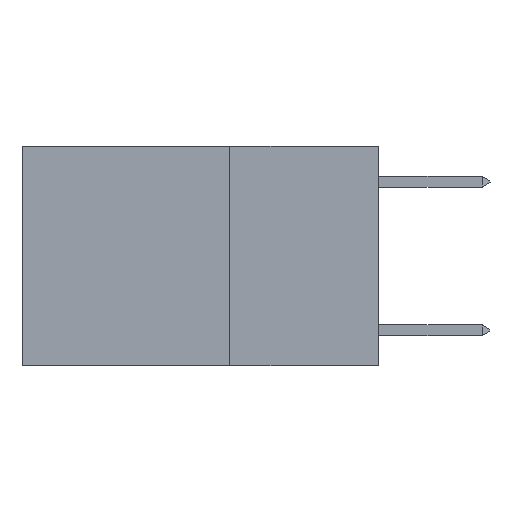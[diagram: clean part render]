
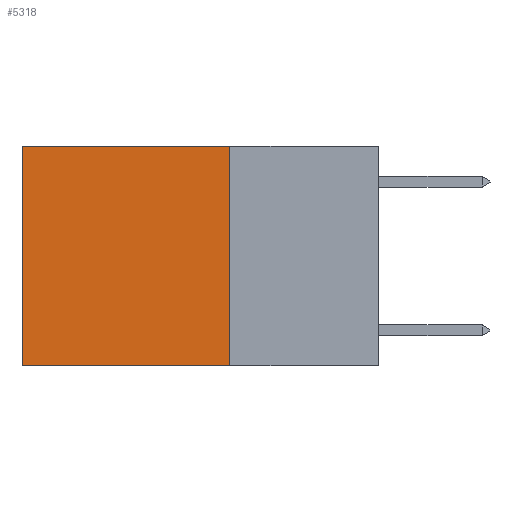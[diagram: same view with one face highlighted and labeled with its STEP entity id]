
A CAD part, left-side view. The second image highlights one B-rep face of the part: STEP entity #5318.
In plain terms, the highlighted planar face has unit normal (-1, 0, 0).
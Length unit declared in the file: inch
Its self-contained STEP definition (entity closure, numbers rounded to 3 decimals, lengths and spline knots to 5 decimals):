
#145 = CARTESIAN_POINT ( 'NONE',  ( 0.2625, 0.6, 0. ) ) ;
#377 = VERTEX_POINT ( 'NONE', #5765 ) ;
#476 = VECTOR ( 'NONE', #7910, 39.37008 ) ;
#865 = CARTESIAN_POINT ( 'NONE',  ( 0.2625, 0.25, 0. ) ) ;
#945 = DIRECTION ( 'NONE',  ( 1., 0., 0. ) ) ;
#957 = DIRECTION ( 'NONE',  ( 0., 1., 0. ) ) ;
#2212 = CARTESIAN_POINT ( 'NONE',  ( 0.2625, 0.6, -0.37 ) ) ;
#2438 = VERTEX_POINT ( 'NONE', #7295 ) ;
#2687 = VECTOR ( 'NONE', #13122, 39.37008 ) ;
#3317 = FACE_OUTER_BOUND ( 'NONE', #9579, .T. ) ;
#3550 = EDGE_CURVE ( 'NONE', #377, #9089, #14127, .T. ) ;
#3612 = ORIENTED_EDGE ( 'NONE', *, *, #13934, .F. ) ;
#4056 = CARTESIAN_POINT ( 'NONE',  ( 0.2625, 0.25, 0. ) ) ;
#4208 = VECTOR ( 'NONE', #7472, 39.37008 ) ;
#4523 = DIRECTION ( 'NONE',  ( 0., 0., -1. ) ) ;
#4984 = ORIENTED_EDGE ( 'NONE', *, *, #5076, .F. ) ;
#5076 = EDGE_CURVE ( 'NONE', #2438, #8968, #8443, .T. ) ;
#5084 = LINE ( 'NONE', #4056, #4208 ) ;
#5301 = CARTESIAN_POINT ( 'NONE',  ( 0.2625, 0.6, 0. ) ) ;
#5318 = ADVANCED_FACE ( 'NONE', ( #3317 ), #15074, .F. ) ;
#5765 = CARTESIAN_POINT ( 'NONE',  ( 0.2625, 0.25, 0. ) ) ;
#7229 = LINE ( 'NONE', #5301, #476 ) ;
#7295 = CARTESIAN_POINT ( 'NONE',  ( 0.2625, 0.25, -0.37 ) ) ;
#7472 = DIRECTION ( 'NONE',  ( 0., 0., -1. ) ) ;
#7910 = DIRECTION ( 'NONE',  ( 0., 0., -1. ) ) ;
#8443 = LINE ( 'NONE', #9407, #2687 ) ;
#8968 = VERTEX_POINT ( 'NONE', #2212 ) ;
#9089 = VERTEX_POINT ( 'NONE', #145 ) ;
#9269 = ORIENTED_EDGE ( 'NONE', *, *, #15321, .T. ) ;
#9407 = CARTESIAN_POINT ( 'NONE',  ( 0.2625, 0.25, -0.37 ) ) ;
#9579 = EDGE_LOOP ( 'NONE', ( #9269, #4984, #3612, #11274 ) ) ;
#11274 = ORIENTED_EDGE ( 'NONE', *, *, #3550, .T. ) ;
#11505 = AXIS2_PLACEMENT_3D ( 'NONE', #865, #945, #4523 ) ;
#12885 = VECTOR ( 'NONE', #957, 39.37008 ) ;
#13122 = DIRECTION ( 'NONE',  ( 0., 1., 0. ) ) ;
#13934 = EDGE_CURVE ( 'NONE', #377, #2438, #5084, .T. ) ;
#14127 = LINE ( 'NONE', #15167, #12885 ) ;
#15074 = PLANE ( 'NONE',  #11505 ) ;
#15167 = CARTESIAN_POINT ( 'NONE',  ( 0.2625, 0.25, 0. ) ) ;
#15321 = EDGE_CURVE ( 'NONE', #9089, #8968, #7229, .T. ) ;
